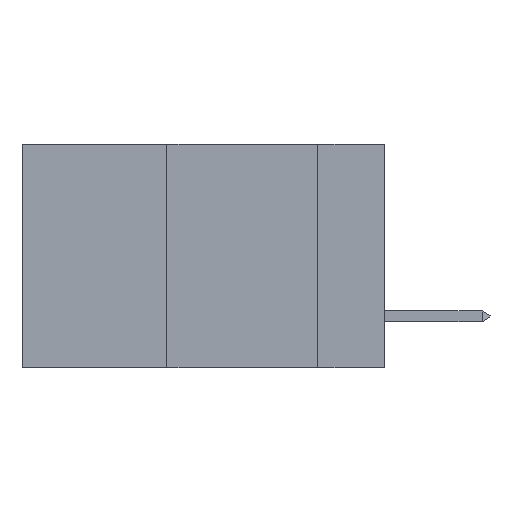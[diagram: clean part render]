
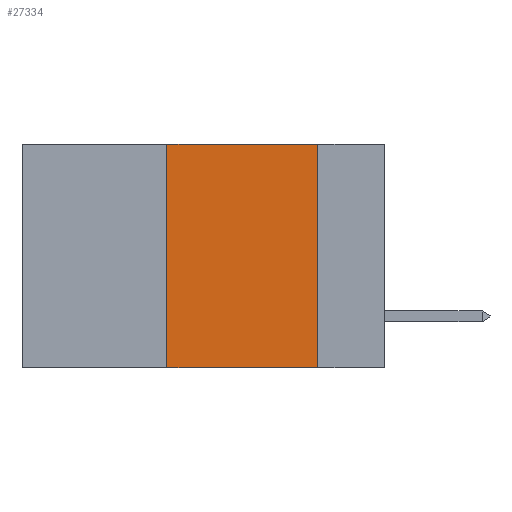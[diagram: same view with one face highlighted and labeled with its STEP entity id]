
A CAD part, left-side view. The second image highlights one B-rep face of the part: STEP entity #27334.
In plain terms, the highlighted planar face has unit normal (-1, 0, 0).
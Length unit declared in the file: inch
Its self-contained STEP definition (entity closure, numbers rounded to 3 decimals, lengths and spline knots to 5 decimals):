
#446 = EDGE_CURVE ( 'NONE', #4400, #46206, #14888, .T. ) ;
#4270 = CARTESIAN_POINT ( 'NONE',  ( 0., 0.36, 0. ) ) ;
#4271 = CARTESIAN_POINT ( 'NONE',  ( 0., 0.6, 0. ) ) ;
#4400 = VERTEX_POINT ( 'NONE', #4270 ) ;
#5176 = DIRECTION ( 'NONE',  ( 0., -1., 0. ) ) ;
#5436 = LINE ( 'NONE', #12507, #41428 ) ;
#6466 = VECTOR ( 'NONE', #5176, 39.37008 ) ;
#6950 = PLANE ( 'NONE',  #8135 ) ;
#8135 = AXIS2_PLACEMENT_3D ( 'NONE', #18044, #14734, #10498 ) ;
#10498 = DIRECTION ( 'NONE',  ( 0., 0., -1. ) ) ;
#12507 = CARTESIAN_POINT ( 'NONE',  ( 0., 0.36, 0. ) ) ;
#14238 = ORIENTED_EDGE ( 'NONE', *, *, #22868, .T. ) ;
#14734 = DIRECTION ( 'NONE',  ( 1., 0., 0. ) ) ;
#14888 = LINE ( 'NONE', #4271, #42711 ) ;
#18044 = CARTESIAN_POINT ( 'NONE',  ( 0., 0.6, 0. ) ) ;
#18656 = DIRECTION ( 'NONE',  ( 0., -1., 0. ) ) ;
#19181 = CARTESIAN_POINT ( 'NONE',  ( 0., 0.36, -0.37 ) ) ;
#22868 = EDGE_CURVE ( 'NONE', #38973, #40371, #30127, .T. ) ;
#23747 = ORIENTED_EDGE ( 'NONE', *, *, #446, .F. ) ;
#25784 = EDGE_LOOP ( 'NONE', ( #40099, #23747, #34078, #14238 ) ) ;
#27306 = CARTESIAN_POINT ( 'NONE',  ( 0., 0.11, 0. ) ) ;
#27334 = ADVANCED_FACE ( 'NONE', ( #42748 ), #6950, .F. ) ;
#27791 = LINE ( 'NONE', #27306, #34202 ) ;
#28555 = CARTESIAN_POINT ( 'NONE',  ( 0., 0.11, -0.37 ) ) ;
#30127 = LINE ( 'NONE', #41883, #6466 ) ;
#34078 = ORIENTED_EDGE ( 'NONE', *, *, #34468, .F. ) ;
#34202 = VECTOR ( 'NONE', #42134, 39.37008 ) ;
#34468 = EDGE_CURVE ( 'NONE', #38973, #4400, #5436, .T. ) ;
#35381 = CARTESIAN_POINT ( 'NONE',  ( 0., 0.11, 0. ) ) ;
#38163 = DIRECTION ( 'NONE',  ( 0., 0., 1. ) ) ;
#38973 = VERTEX_POINT ( 'NONE', #19181 ) ;
#40099 = ORIENTED_EDGE ( 'NONE', *, *, #41829, .F. ) ;
#40371 = VERTEX_POINT ( 'NONE', #28555 ) ;
#41428 = VECTOR ( 'NONE', #38163, 39.37008 ) ;
#41829 = EDGE_CURVE ( 'NONE', #46206, #40371, #27791, .T. ) ;
#41883 = CARTESIAN_POINT ( 'NONE',  ( 0., 0.6, -0.37 ) ) ;
#42134 = DIRECTION ( 'NONE',  ( 0., 0., -1. ) ) ;
#42711 = VECTOR ( 'NONE', #18656, 39.37008 ) ;
#42748 = FACE_OUTER_BOUND ( 'NONE', #25784, .T. ) ;
#46206 = VERTEX_POINT ( 'NONE', #35381 ) ;
